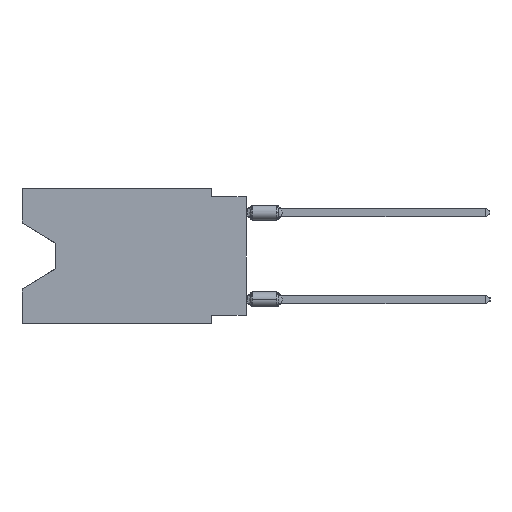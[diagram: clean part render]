
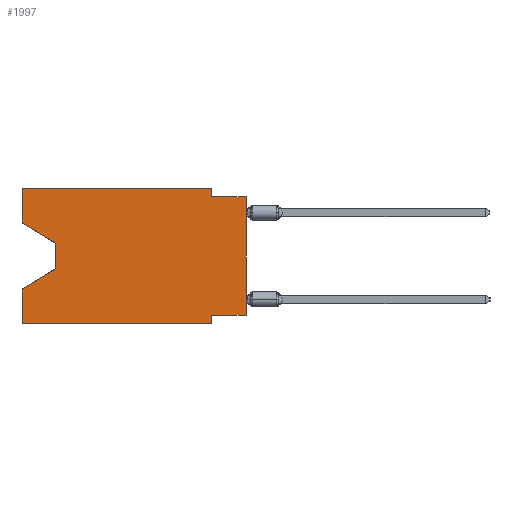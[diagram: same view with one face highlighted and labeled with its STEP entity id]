
A CAD part, left-side view. The second image highlights one B-rep face of the part: STEP entity #1997.
In plain terms, the highlighted planar face has unit normal (-1, 0, 0).
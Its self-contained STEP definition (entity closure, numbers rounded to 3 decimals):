
#332 = DIRECTION ( 'NONE',  ( 0., 0., 1. ) ) ;
#670 = CARTESIAN_POINT ( 'NONE',  ( 0., 16.383, -2.546 ) ) ;
#852 = VECTOR ( 'NONE', #11324, 1000. ) ;
#1997 = ADVANCED_FACE ( 'NONE', ( #21353 ), #28139, .F. ) ;
#2040 = EDGE_CURVE ( 'NONE', #23043, #22200, #17906, .T. ) ;
#2377 = DIRECTION ( 'NONE',  ( 0., 0., -1. ) ) ;
#2555 = ORIENTED_EDGE ( 'NONE', *, *, #7951, .T. ) ;
#2705 = ORIENTED_EDGE ( 'NONE', *, *, #22020, .F. ) ;
#4236 = VECTOR ( 'NONE', #34564, 1000. ) ;
#4464 = LINE ( 'NONE', #22457, #47739 ) ;
#4850 = LINE ( 'NONE', #41297, #5539 ) ;
#5539 = VECTOR ( 'NONE', #26484, 1000. ) ;
#6337 = LINE ( 'NONE', #28694, #47424 ) ;
#6416 = DIRECTION ( 'NONE',  ( 0., -1., 0. ) ) ;
#6502 = DIRECTION ( 'NONE',  ( 1., 0., 0. ) ) ;
#6950 = CARTESIAN_POINT ( 'NONE',  ( 0., 2.54, -9.906 ) ) ;
#7423 = EDGE_LOOP ( 'NONE', ( #2555, #17087, #35879, #28673, #34023, #2705, #8751, #31433, #8489, #33048, #9570, #22313 ) ) ;
#7442 = LINE ( 'NONE', #22522, #36917 ) ;
#7951 = EDGE_CURVE ( 'NONE', #40671, #33105, #36649, .T. ) ;
#8489 = ORIENTED_EDGE ( 'NONE', *, *, #47279, .F. ) ;
#8751 = ORIENTED_EDGE ( 'NONE', *, *, #13103, .F. ) ;
#8754 = DIRECTION ( 'NONE',  ( 0., 0., 1. ) ) ;
#8819 = CARTESIAN_POINT ( 'NONE',  ( 0., 0., -0.635 ) ) ;
#8908 = VERTEX_POINT ( 'NONE', #34993 ) ;
#9570 = ORIENTED_EDGE ( 'NONE', *, *, #33060, .F. ) ;
#10052 = CARTESIAN_POINT ( 'NONE',  ( 0., 2.54, -9.906 ) ) ;
#10143 = CARTESIAN_POINT ( 'NONE',  ( 0., 2.54, 0. ) ) ;
#11324 = DIRECTION ( 'NONE',  ( 0., 0., -1. ) ) ;
#12509 = CARTESIAN_POINT ( 'NONE',  ( 0., 2.54, -0.635 ) ) ;
#13103 = EDGE_CURVE ( 'NONE', #8908, #27678, #43281, .T. ) ;
#13113 = CARTESIAN_POINT ( 'NONE',  ( 0., 16.383, 0. ) ) ;
#13158 = LINE ( 'NONE', #8819, #4236 ) ;
#13573 = VERTEX_POINT ( 'NONE', #13113 ) ;
#14321 = CARTESIAN_POINT ( 'NONE',  ( 0., 16.383, -2.546 ) ) ;
#14439 = CARTESIAN_POINT ( 'NONE',  ( 0., 16.383, -9.906 ) ) ;
#15090 = CARTESIAN_POINT ( 'NONE',  ( 0., 0., -0.635 ) ) ;
#15477 = VERTEX_POINT ( 'NONE', #46681 ) ;
#16373 = VECTOR ( 'NONE', #41374, 1000. ) ;
#16453 = EDGE_CURVE ( 'NONE', #40671, #13573, #4464, .T. ) ;
#17087 = ORIENTED_EDGE ( 'NONE', *, *, #17666, .T. ) ;
#17666 = EDGE_CURVE ( 'NONE', #33105, #29437, #7442, .T. ) ;
#17906 = LINE ( 'NONE', #10143, #28546 ) ;
#19132 = DIRECTION ( 'NONE',  ( 0., 0., -1. ) ) ;
#19249 = CARTESIAN_POINT ( 'NONE',  ( 0., 2.54, 0. ) ) ;
#21353 = FACE_OUTER_BOUND ( 'NONE', #7423, .T. ) ;
#21400 = EDGE_CURVE ( 'NONE', #41134, #15477, #27213, .T. ) ;
#22020 = EDGE_CURVE ( 'NONE', #27678, #42540, #26379, .T. ) ;
#22200 = VERTEX_POINT ( 'NONE', #12509 ) ;
#22313 = ORIENTED_EDGE ( 'NONE', *, *, #16453, .F. ) ;
#22457 = CARTESIAN_POINT ( 'NONE',  ( 0., 16.383, 0. ) ) ;
#22522 = CARTESIAN_POINT ( 'NONE',  ( 0., 13.97, -4.013 ) ) ;
#23043 = VERTEX_POINT ( 'NONE', #19249 ) ;
#23529 = VECTOR ( 'NONE', #6416, 1000. ) ;
#24353 = DIRECTION ( 'NONE',  ( 0., 0., 1. ) ) ;
#26379 = LINE ( 'NONE', #6950, #852 ) ;
#26484 = DIRECTION ( 'NONE',  ( 0., 0.855, -0.519 ) ) ;
#26712 = VECTOR ( 'NONE', #46688, 1000. ) ;
#27192 = VERTEX_POINT ( 'NONE', #15090 ) ;
#27213 = LINE ( 'NONE', #42017, #32926 ) ;
#27566 = CARTESIAN_POINT ( 'NONE',  ( 0., 16.383, -9.906 ) ) ;
#27678 = VERTEX_POINT ( 'NONE', #43496 ) ;
#28139 = PLANE ( 'NONE',  #36301 ) ;
#28481 = EDGE_CURVE ( 'NONE', #41134, #42540, #32645, .T. ) ;
#28546 = VECTOR ( 'NONE', #46586, 1000. ) ;
#28673 = ORIENTED_EDGE ( 'NONE', *, *, #21400, .F. ) ;
#28694 = CARTESIAN_POINT ( 'NONE',  ( 0., 0., 0. ) ) ;
#29437 = VERTEX_POINT ( 'NONE', #37368 ) ;
#30331 = VECTOR ( 'NONE', #41252, 1000. ) ;
#31084 = CARTESIAN_POINT ( 'NONE',  ( 0., 13.97, -4.013 ) ) ;
#31433 = ORIENTED_EDGE ( 'NONE', *, *, #31635, .T. ) ;
#31635 = EDGE_CURVE ( 'NONE', #8908, #27192, #6337, .T. ) ;
#31807 = EDGE_CURVE ( 'NONE', #29437, #15477, #4850, .T. ) ;
#32645 = LINE ( 'NONE', #14439, #23529 ) ;
#32926 = VECTOR ( 'NONE', #8754, 1000. ) ;
#33048 = ORIENTED_EDGE ( 'NONE', *, *, #2040, .F. ) ;
#33060 = EDGE_CURVE ( 'NONE', #13573, #23043, #42268, .T. ) ;
#33105 = VERTEX_POINT ( 'NONE', #31084 ) ;
#33599 = CARTESIAN_POINT ( 'NONE',  ( 0., 16.383, 0. ) ) ;
#34023 = ORIENTED_EDGE ( 'NONE', *, *, #28481, .T. ) ;
#34564 = DIRECTION ( 'NONE',  ( 0., -1., 0. ) ) ;
#34993 = CARTESIAN_POINT ( 'NONE',  ( 0., 0., -9.271 ) ) ;
#35879 = ORIENTED_EDGE ( 'NONE', *, *, #31807, .T. ) ;
#36301 = AXIS2_PLACEMENT_3D ( 'NONE', #42944, #6502, #2377 ) ;
#36649 = LINE ( 'NONE', #14321, #30331 ) ;
#36917 = VECTOR ( 'NONE', #19132, 1000. ) ;
#37368 = CARTESIAN_POINT ( 'NONE',  ( 0., 13.97, -5.893 ) ) ;
#40671 = VERTEX_POINT ( 'NONE', #670 ) ;
#41134 = VERTEX_POINT ( 'NONE', #27566 ) ;
#41252 = DIRECTION ( 'NONE',  ( 0., -0.855, -0.519 ) ) ;
#41297 = CARTESIAN_POINT ( 'NONE',  ( 0., 13.97, -5.893 ) ) ;
#41374 = DIRECTION ( 'NONE',  ( 0., -1., 0. ) ) ;
#42017 = CARTESIAN_POINT ( 'NONE',  ( 0., 16.383, 0. ) ) ;
#42268 = LINE ( 'NONE', #33599, #16373 ) ;
#42540 = VERTEX_POINT ( 'NONE', #10052 ) ;
#42567 = CARTESIAN_POINT ( 'NONE',  ( 0., 0., -9.271 ) ) ;
#42944 = CARTESIAN_POINT ( 'NONE',  ( 0., 16.383, 0. ) ) ;
#43281 = LINE ( 'NONE', #42567, #26712 ) ;
#43496 = CARTESIAN_POINT ( 'NONE',  ( 0., 2.54, -9.271 ) ) ;
#46586 = DIRECTION ( 'NONE',  ( 0., 0., -1. ) ) ;
#46681 = CARTESIAN_POINT ( 'NONE',  ( 0., 16.383, -7.36 ) ) ;
#46688 = DIRECTION ( 'NONE',  ( 0., 1., 0. ) ) ;
#47279 = EDGE_CURVE ( 'NONE', #22200, #27192, #13158, .T. ) ;
#47424 = VECTOR ( 'NONE', #24353, 1000. ) ;
#47739 = VECTOR ( 'NONE', #332, 1000. ) ;
